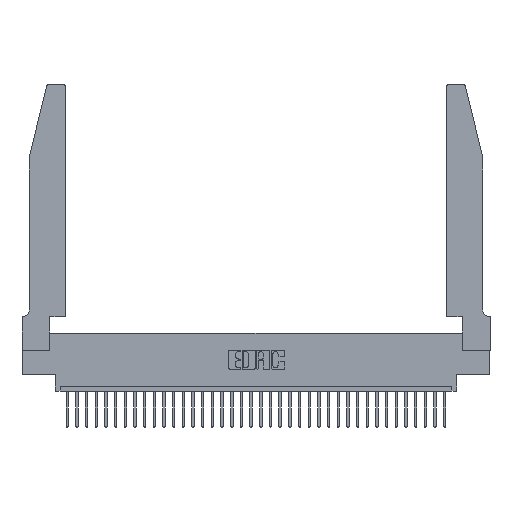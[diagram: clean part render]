
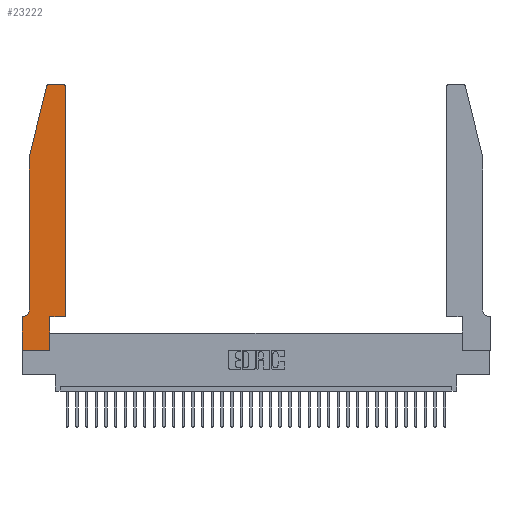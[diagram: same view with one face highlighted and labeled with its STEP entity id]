
A CAD part, top view. The second image highlights one B-rep face of the part: STEP entity #23222.
In plain terms, the highlighted planar face has unit normal (0, 0, 1).
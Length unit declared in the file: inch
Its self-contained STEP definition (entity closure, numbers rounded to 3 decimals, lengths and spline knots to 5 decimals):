
#190 = CARTESIAN_POINT ( 'NONE',  ( 0., 0.35, 0.37 ) ) ;
#245 = CARTESIAN_POINT ( 'NONE',  ( 0.0055, 0.42, 0.37 ) ) ;
#606 = LINE ( 'NONE', #18509, #7462 ) ;
#753 = CARTESIAN_POINT ( 'NONE',  ( 0., 0.35, 0.37 ) ) ;
#759 = DIRECTION ( 'NONE',  ( 0., 0., 1. ) ) ;
#1348 = CIRCLE ( 'NONE', #34334, 0.03 ) ;
#1415 = CARTESIAN_POINT ( 'NONE',  ( 0.2865, 0.35, 0.37 ) ) ;
#1735 = VERTEX_POINT ( 'NONE', #21795 ) ;
#2262 = DIRECTION ( 'NONE',  ( 0., -1., 0. ) ) ;
#2760 = ORIENTED_EDGE ( 'NONE', *, *, #10688, .T. ) ;
#2977 = CARTESIAN_POINT ( 'NONE',  ( 0.2865, 0., 0.37 ) ) ;
#3159 = DIRECTION ( 'NONE',  ( 0., 0., 1. ) ) ;
#3526 = CARTESIAN_POINT ( 'NONE',  ( 0.2605, 2.75, 0.37 ) ) ;
#3588 = DIRECTION ( 'NONE',  ( 0., 0., 1. ) ) ;
#3877 = DIRECTION ( 'NONE',  ( 0., 1., 0. ) ) ;
#4254 = CARTESIAN_POINT ( 'NONE',  ( 0.2865, 0.35, 0.37 ) ) ;
#4622 = DIRECTION ( 'NONE',  ( -0.239, -0.971, 0. ) ) ;
#5023 = EDGE_CURVE ( 'NONE', #7620, #34285, #34037, .T. ) ;
#5928 = DIRECTION ( 'NONE',  ( 1., 0., 0. ) ) ;
#6382 = DIRECTION ( 'NONE',  ( 1., 0., 0. ) ) ;
#7055 = EDGE_CURVE ( 'NONE', #34285, #33615, #15521, .T. ) ;
#7079 = DIRECTION ( 'NONE',  ( 1., 0., 0. ) ) ;
#7462 = VECTOR ( 'NONE', #2262, 39.37008 ) ;
#7620 = VERTEX_POINT ( 'NONE', #1415 ) ;
#7636 = LINE ( 'NONE', #3526, #21642 ) ;
#8255 = DIRECTION ( 'NONE',  ( -1., 0., 0. ) ) ;
#8268 = EDGE_CURVE ( 'NONE', #11142, #26969, #22698, .T. ) ;
#8432 = EDGE_CURVE ( 'NONE', #22134, #32717, #9102, .T. ) ;
#8781 = ORIENTED_EDGE ( 'NONE', *, *, #8268, .T. ) ;
#8835 = DIRECTION ( 'NONE',  ( 1., 0., 0. ) ) ;
#9102 = LINE ( 'NONE', #20352, #15491 ) ;
#9277 = EDGE_CURVE ( 'NONE', #23206, #11142, #1348, .T. ) ;
#9872 = EDGE_CURVE ( 'NONE', #1735, #29791, #12398, .T. ) ;
#10652 = CARTESIAN_POINT ( 'NONE',  ( 0.0755, 0.42, 0.37 ) ) ;
#10683 = CARTESIAN_POINT ( 'NONE',  ( 0.25487, 2.72718, 0.37 ) ) ;
#10688 = EDGE_CURVE ( 'NONE', #19863, #23206, #7636, .T. ) ;
#11142 = VERTEX_POINT ( 'NONE', #10683 ) ;
#11323 = DIRECTION ( 'NONE',  ( 0., 1., 0. ) ) ;
#11618 = EDGE_CURVE ( 'NONE', #29791, #22134, #30128, .T. ) ;
#12014 = CARTESIAN_POINT ( 'NONE',  ( 0.4505, 2.72, 0.37 ) ) ;
#12065 = CARTESIAN_POINT ( 'NONE',  ( 0.4205, 2.72, 0.37 ) ) ;
#12398 = LINE ( 'NONE', #29661, #19535 ) ;
#12866 = ORIENTED_EDGE ( 'NONE', *, *, #32326, .T. ) ;
#14074 = FACE_OUTER_BOUND ( 'NONE', #19328, .T. ) ;
#14229 = ORIENTED_EDGE ( 'NONE', *, *, #9277, .T. ) ;
#15183 = ORIENTED_EDGE ( 'NONE', *, *, #11618, .T. ) ;
#15491 = VECTOR ( 'NONE', #7079, 39.37008 ) ;
#15521 = LINE ( 'NONE', #24982, #23592 ) ;
#16657 = CARTESIAN_POINT ( 'NONE',  ( 0.4205, 2.75, 0.37 ) ) ;
#16719 = CARTESIAN_POINT ( 'NONE',  ( 0.0755, 2., 0.37 ) ) ;
#17486 = ORIENTED_EDGE ( 'NONE', *, *, #22886, .T. ) ;
#18135 = ORIENTED_EDGE ( 'NONE', *, *, #22766, .T. ) ;
#18509 = CARTESIAN_POINT ( 'NONE',  ( 0.0755, 2., 0.37 ) ) ;
#19042 = CARTESIAN_POINT ( 'NONE',  ( 0.4505, 0.35, 0.37 ) ) ;
#19120 = CIRCLE ( 'NONE', #25411, 0.03 ) ;
#19328 = EDGE_LOOP ( 'NONE', ( #2760, #14229, #8781, #20292, #18135, #19998, #15183, #35266, #12866, #32378, #27147, #17486 ) ) ;
#19365 = DIRECTION ( 'NONE',  ( 0., 0., -1. ) ) ;
#19535 = VECTOR ( 'NONE', #29775, 39.37008 ) ;
#19863 = VERTEX_POINT ( 'NONE', #16657 ) ;
#19998 = ORIENTED_EDGE ( 'NONE', *, *, #9872, .T. ) ;
#20110 = VECTOR ( 'NONE', #4622, 39.37008 ) ;
#20292 = ORIENTED_EDGE ( 'NONE', *, *, #26194, .T. ) ;
#20352 = CARTESIAN_POINT ( 'NONE',  ( 0., 0., 0.37 ) ) ;
#21105 = CARTESIAN_POINT ( 'NONE',  ( 0.0755, 2., 0.37 ) ) ;
#21642 = VECTOR ( 'NONE', #25317, 39.37008 ) ;
#21795 = CARTESIAN_POINT ( 'NONE',  ( 0.0055, 0.35, 0.37 ) ) ;
#22134 = VERTEX_POINT ( 'NONE', #27124 ) ;
#22698 = LINE ( 'NONE', #21105, #20110 ) ;
#22766 = EDGE_CURVE ( 'NONE', #33889, #1735, #27698, .T. ) ;
#22886 = EDGE_CURVE ( 'NONE', #33615, #19863, #19120, .T. ) ;
#22918 = VECTOR ( 'NONE', #32679, 39.37008 ) ;
#22928 = VECTOR ( 'NONE', #29697, 39.37008 ) ;
#23206 = VERTEX_POINT ( 'NONE', #27448 ) ;
#23222 = ADVANCED_FACE ( 'NONE', ( #14074 ), #32829, .T. ) ;
#23584 = AXIS2_PLACEMENT_3D ( 'NONE', #245, #19365, #8255 ) ;
#23592 = VECTOR ( 'NONE', #11323, 39.37008 ) ;
#24982 = CARTESIAN_POINT ( 'NONE',  ( 0.4505, 0.35, 0.37 ) ) ;
#25317 = DIRECTION ( 'NONE',  ( -1., 0., 0. ) ) ;
#25411 = AXIS2_PLACEMENT_3D ( 'NONE', #12065, #3588, #8835 ) ;
#25516 = CARTESIAN_POINT ( 'NONE',  ( 0.284, 2.72, 0.37 ) ) ;
#26194 = EDGE_CURVE ( 'NONE', #26969, #33889, #606, .T. ) ;
#26491 = VECTOR ( 'NONE', #3877, 39.37008 ) ;
#26732 = CARTESIAN_POINT ( 'NONE',  ( 0., 0., 0.37 ) ) ;
#26969 = VERTEX_POINT ( 'NONE', #16719 ) ;
#27124 = CARTESIAN_POINT ( 'NONE',  ( 0., 0., 0.37 ) ) ;
#27147 = ORIENTED_EDGE ( 'NONE', *, *, #7055, .T. ) ;
#27448 = CARTESIAN_POINT ( 'NONE',  ( 0.284, 2.75, 0.37 ) ) ;
#27698 = CIRCLE ( 'NONE', #23584, 0.07 ) ;
#29661 = CARTESIAN_POINT ( 'NONE',  ( 0.0755, 0.35, 0.37 ) ) ;
#29697 = DIRECTION ( 'NONE',  ( 0., -1., 0. ) ) ;
#29775 = DIRECTION ( 'NONE',  ( -1., 0., 0. ) ) ;
#29791 = VERTEX_POINT ( 'NONE', #753 ) ;
#30128 = LINE ( 'NONE', #26732, #22928 ) ;
#31203 = LINE ( 'NONE', #4254, #26491 ) ;
#32052 = AXIS2_PLACEMENT_3D ( 'NONE', #190, #3159, #5928 ) ;
#32326 = EDGE_CURVE ( 'NONE', #32717, #7620, #31203, .T. ) ;
#32378 = ORIENTED_EDGE ( 'NONE', *, *, #5023, .T. ) ;
#32679 = DIRECTION ( 'NONE',  ( 1., 0., 0. ) ) ;
#32717 = VERTEX_POINT ( 'NONE', #2977 ) ;
#32829 = PLANE ( 'NONE',  #32052 ) ;
#33615 = VERTEX_POINT ( 'NONE', #12014 ) ;
#33889 = VERTEX_POINT ( 'NONE', #10652 ) ;
#34037 = LINE ( 'NONE', #19042, #22918 ) ;
#34285 = VERTEX_POINT ( 'NONE', #35176 ) ;
#34334 = AXIS2_PLACEMENT_3D ( 'NONE', #25516, #759, #6382 ) ;
#35176 = CARTESIAN_POINT ( 'NONE',  ( 0.4505, 0.35, 0.37 ) ) ;
#35266 = ORIENTED_EDGE ( 'NONE', *, *, #8432, .T. ) ;
